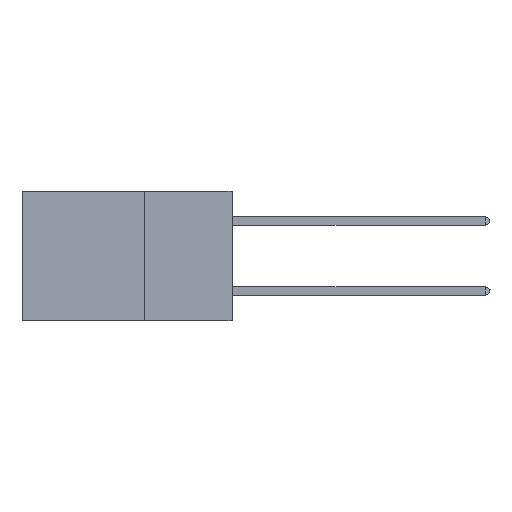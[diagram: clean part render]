
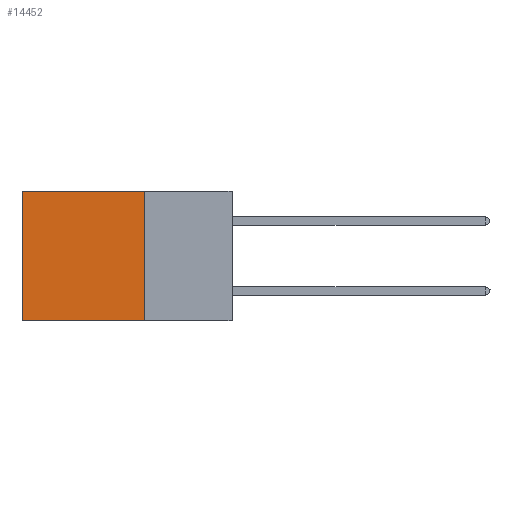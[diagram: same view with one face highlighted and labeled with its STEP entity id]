
A CAD part, left-side view. The second image highlights one B-rep face of the part: STEP entity #14452.
In plain terms, the highlighted planar face has unit normal (-1, 0, 0).
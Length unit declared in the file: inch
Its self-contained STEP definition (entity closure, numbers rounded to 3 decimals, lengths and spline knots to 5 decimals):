
#425 = AXIS2_PLACEMENT_3D ( 'NONE', #35144, #37697, #34949 ) ;
#452 = CARTESIAN_POINT ( 'NONE',  ( 0.2875, 0.25, -0.37 ) ) ;
#580 = EDGE_LOOP ( 'NONE', ( #35028, #18539, #14047, #18019 ) ) ;
#1337 = EDGE_CURVE ( 'NONE', #8281, #28304, #31084, .T. ) ;
#2131 = FACE_OUTER_BOUND ( 'NONE', #580, .T. ) ;
#2276 = DIRECTION ( 'NONE',  ( 0., 1., 0. ) ) ;
#4416 = DIRECTION ( 'NONE',  ( 0., 0., -1. ) ) ;
#8281 = VERTEX_POINT ( 'NONE', #15111 ) ;
#8489 = CARTESIAN_POINT ( 'NONE',  ( 0.2875, 0.25, -0.37 ) ) ;
#8598 = VECTOR ( 'NONE', #30012, 39.37008 ) ;
#10941 = VERTEX_POINT ( 'NONE', #17910 ) ;
#11109 = CARTESIAN_POINT ( 'NONE',  ( 0.2875, 0.6, -0.37 ) ) ;
#14047 = ORIENTED_EDGE ( 'NONE', *, *, #18221, .F. ) ;
#14452 = ADVANCED_FACE ( 'NONE', ( #2131 ), #28564, .F. ) ;
#15017 = EDGE_CURVE ( 'NONE', #18199, #28304, #26185, .T. ) ;
#15111 = CARTESIAN_POINT ( 'NONE',  ( 0.2875, 0.6, 0. ) ) ;
#15198 = VECTOR ( 'NONE', #4416, 39.37008 ) ;
#17910 = CARTESIAN_POINT ( 'NONE',  ( 0.2875, 0.25, 0. ) ) ;
#18019 = ORIENTED_EDGE ( 'NONE', *, *, #19623, .T. ) ;
#18199 = VERTEX_POINT ( 'NONE', #452 ) ;
#18221 = EDGE_CURVE ( 'NONE', #10941, #18199, #18542, .T. ) ;
#18338 = CARTESIAN_POINT ( 'NONE',  ( 0.2875, 0.25, 0. ) ) ;
#18479 = VECTOR ( 'NONE', #2276, 39.37008 ) ;
#18539 = ORIENTED_EDGE ( 'NONE', *, *, #15017, .F. ) ;
#18542 = LINE ( 'NONE', #18338, #8598 ) ;
#19623 = EDGE_CURVE ( 'NONE', #10941, #8281, #36017, .T. ) ;
#26185 = LINE ( 'NONE', #8489, #18479 ) ;
#27281 = DIRECTION ( 'NONE',  ( 0., 1., 0. ) ) ;
#27371 = CARTESIAN_POINT ( 'NONE',  ( 0.2875, 0.6, 0. ) ) ;
#28304 = VERTEX_POINT ( 'NONE', #11109 ) ;
#28564 = PLANE ( 'NONE',  #425 ) ;
#30012 = DIRECTION ( 'NONE',  ( 0., 0., -1. ) ) ;
#30212 = CARTESIAN_POINT ( 'NONE',  ( 0.2875, 0.25, 0. ) ) ;
#31084 = LINE ( 'NONE', #27371, #15198 ) ;
#34099 = VECTOR ( 'NONE', #27281, 39.37008 ) ;
#34949 = DIRECTION ( 'NONE',  ( 0., 0., -1. ) ) ;
#35028 = ORIENTED_EDGE ( 'NONE', *, *, #1337, .T. ) ;
#35144 = CARTESIAN_POINT ( 'NONE',  ( 0.2875, 0.25, 0. ) ) ;
#36017 = LINE ( 'NONE', #30212, #34099 ) ;
#37697 = DIRECTION ( 'NONE',  ( 1., 0., 0. ) ) ;
